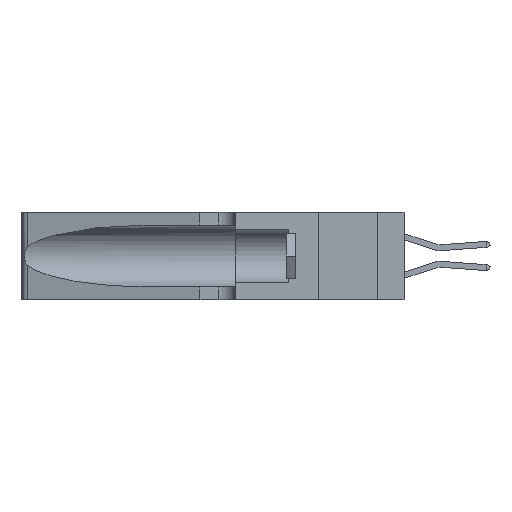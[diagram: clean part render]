
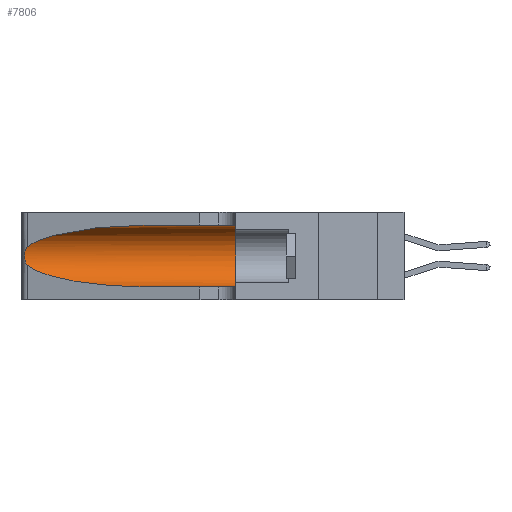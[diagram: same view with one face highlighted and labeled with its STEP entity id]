
A CAD part, left-side view. The second image highlights one B-rep face of the part: STEP entity #7806.
In plain terms, the highlighted cylindrical face has radius 3.308 mm (diameter 6.617 mm), a partial arc.
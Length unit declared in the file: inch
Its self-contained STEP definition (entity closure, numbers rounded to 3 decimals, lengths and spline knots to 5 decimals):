
#732 = DIRECTION ( 'NONE',  ( 0., 1., 0. ) ) ;
#754 = CARTESIAN_POINT ( 'NONE',  ( 0.1305, 0.72297, 0.05475 ) ) ;
#966 = CARTESIAN_POINT ( 'NONE',  ( 0.1305, 0.35, 0.31525 ) ) ;
#1230 = EDGE_CURVE ( 'NONE', #27923, #3265, #6271, .T. ) ;
#1282 = EDGE_CURVE ( 'NONE', #16083, #21831, #34458, .T. ) ;
#2385 =( BOUNDED_CURVE ( )  B_SPLINE_CURVE ( 3, ( #18711, #34994, #7792, #26921 ),
 .UNSPECIFIED., .F., .F. ) 
 B_SPLINE_CURVE_WITH_KNOTS ( ( 4, 4 ),
 ( 1.5708, 2.84003 ),
 .UNSPECIFIED. ) 
 CURVE ( )  GEOMETRIC_REPRESENTATION_ITEM ( )  RATIONAL_B_SPLINE_CURVE ( ( 1., 0.87, 0.87, 1. ) ) 
 REPRESENTATION_ITEM ( '' )  );
#3265 = VERTEX_POINT ( 'NONE', #14024 ) ;
#3901 = CARTESIAN_POINT ( 'NONE',  ( 0.25787, 1.23484, 0.2124 ) ) ;
#4734 = FACE_OUTER_BOUND ( 'NONE', #21937, .T. ) ;
#5455 = VERTEX_POINT ( 'NONE', #12333 ) ;
#5856 = ORIENTED_EDGE ( 'NONE', *, *, #14432, .T. ) ;
#6271 = LINE ( 'NONE', #33257, #12758 ) ;
#6615 = CARTESIAN_POINT ( 'NONE',  ( 0.26018, 1.23835, 0.19895 ) ) ;
#7516 = EDGE_CURVE ( 'NONE', #21831, #3265, #35022, .T. ) ;
#7792 = CARTESIAN_POINT ( 'NONE',  ( 0.2373, 1.15595, 0.28018 ) ) ;
#7806 = ADVANCED_FACE ( 'NONE', ( #4734 ), #18426, .F. ) ;
#8957 = CARTESIAN_POINT ( 'NONE',  ( 0.1305, 1.61858, 0.31525 ) ) ;
#9078 = ORIENTED_EDGE ( 'NONE', *, *, #21233, .T. ) ;
#9411 = CARTESIAN_POINT ( 'NONE',  ( 0.26075, 1.23896, 0.178 ) ) ;
#9803 = CARTESIAN_POINT ( 'NONE',  ( 0.25487, 1.22718, 0.14631 ) ) ;
#12179 = CARTESIAN_POINT ( 'NONE',  ( 0.25856, 1.23593, 0.16098 ) ) ;
#12333 = CARTESIAN_POINT ( 'NONE',  ( 0.25487, 1.22718, 0.22369 ) ) ;
#12522 = B_SPLINE_CURVE_WITH_KNOTS ( 'NONE', 3,
 ( #33800, #14803, #20250, #3901, #23009, #6615, #25760, #9411, #28487, #12179, #31210, #14924, #33919, #17688 ),
 .UNSPECIFIED., .F., .F.,
 ( 4, 2, 2, 2, 2, 2, 4 ),
 ( 0., 0.00027, 0.00053, 0.00107, 0.0016, 0.00187, 0.00214 ),
 .UNSPECIFIED. ) ;
#12758 = VECTOR ( 'NONE', #19810, 39.37008 ) ;
#14024 = CARTESIAN_POINT ( 'NONE',  ( 0.1305, 0.35, 0.05475 ) ) ;
#14432 = EDGE_CURVE ( 'NONE', #16083, #5455, #2385, .T. ) ;
#14803 = CARTESIAN_POINT ( 'NONE',  ( 0.25555, 1.22994, 0.2215 ) ) ;
#14924 = CARTESIAN_POINT ( 'NONE',  ( 0.25639, 1.23186, 0.15144 ) ) ;
#15483 = DIRECTION ( 'NONE',  ( 0., 0., -1. ) ) ;
#16035 = ORIENTED_EDGE ( 'NONE', *, *, #17058, .T. ) ;
#16083 = VERTEX_POINT ( 'NONE', #19166 ) ;
#16690 = ORIENTED_EDGE ( 'NONE', *, *, #1282, .F. ) ;
#16814 = ORIENTED_EDGE ( 'NONE', *, *, #1230, .T. ) ;
#17058 = EDGE_CURVE ( 'NONE', #26505, #27923, #31476, .T. ) ;
#17178 = CARTESIAN_POINT ( 'NONE',  ( 0.1305, 0.35, 0.185 ) ) ;
#17688 = CARTESIAN_POINT ( 'NONE',  ( 0.25487, 1.22718, 0.14631 ) ) ;
#17956 = CARTESIAN_POINT ( 'NONE',  ( 0.18966, 0.96281, 0.05475 ) ) ;
#18426 = CYLINDRICAL_SURFACE ( 'NONE', #27616, 0.13025 ) ;
#18711 = CARTESIAN_POINT ( 'NONE',  ( 0.1305, 0.72297, 0.31525 ) ) ;
#19166 = CARTESIAN_POINT ( 'NONE',  ( 0.1305, 0.72297, 0.31525 ) ) ;
#19810 = DIRECTION ( 'NONE',  ( 0., -1., 0. ) ) ;
#19868 = DIRECTION ( 'NONE',  ( 0., 0., 1. ) ) ;
#20250 = CARTESIAN_POINT ( 'NONE',  ( 0.25639, 1.23184, 0.21858 ) ) ;
#21233 = EDGE_CURVE ( 'NONE', #5455, #26505, #12522, .T. ) ;
#21831 = VERTEX_POINT ( 'NONE', #966 ) ;
#21937 = EDGE_LOOP ( 'NONE', ( #5856, #9078, #16035, #16814, #25113, #16690 ) ) ;
#23009 = CARTESIAN_POINT ( 'NONE',  ( 0.25854, 1.2359, 0.20912 ) ) ;
#23416 = CARTESIAN_POINT ( 'NONE',  ( 0.2373, 1.15595, 0.08982 ) ) ;
#25113 = ORIENTED_EDGE ( 'NONE', *, *, #7516, .F. ) ;
#25423 = DIRECTION ( 'NONE',  ( 0., -1., 0. ) ) ;
#25530 = VECTOR ( 'NONE', #25423, 39.37008 ) ;
#25760 = CARTESIAN_POINT ( 'NONE',  ( 0.26075, 1.23896, 0.19203 ) ) ;
#26319 = DIRECTION ( 'NONE',  ( 0., -1., 0. ) ) ;
#26505 = VERTEX_POINT ( 'NONE', #32299 ) ;
#26921 = CARTESIAN_POINT ( 'NONE',  ( 0.25487, 1.22718, 0.22369 ) ) ;
#27616 = AXIS2_PLACEMENT_3D ( 'NONE', #31754, #26319, #15483 ) ;
#27923 = VERTEX_POINT ( 'NONE', #754 ) ;
#28487 = CARTESIAN_POINT ( 'NONE',  ( 0.26017, 1.23833, 0.17102 ) ) ;
#28872 = CARTESIAN_POINT ( 'NONE',  ( 0.1305, 0.72297, 0.05475 ) ) ;
#30110 = AXIS2_PLACEMENT_3D ( 'NONE', #17178, #732, #19868 ) ;
#31210 = CARTESIAN_POINT ( 'NONE',  ( 0.25789, 1.23486, 0.15765 ) ) ;
#31476 =( BOUNDED_CURVE ( )  B_SPLINE_CURVE ( 3, ( #9803, #23416, #17956, #28872 ),
 .UNSPECIFIED., .F., .T. ) 
 B_SPLINE_CURVE_WITH_KNOTS ( ( 4, 4 ),
 ( 3.44316, 4.71239 ),
 .UNSPECIFIED. ) 
 CURVE ( )  GEOMETRIC_REPRESENTATION_ITEM ( )  RATIONAL_B_SPLINE_CURVE ( ( 1., 0.87, 0.87, 1. ) ) 
 REPRESENTATION_ITEM ( '' )  );
#31754 = CARTESIAN_POINT ( 'NONE',  ( 0.1305, 1.61858, 0.185 ) ) ;
#32299 = CARTESIAN_POINT ( 'NONE',  ( 0.25487, 1.22718, 0.14631 ) ) ;
#33257 = CARTESIAN_POINT ( 'NONE',  ( 0.1305, 1.61858, 0.05475 ) ) ;
#33800 = CARTESIAN_POINT ( 'NONE',  ( 0.25487, 1.22718, 0.22369 ) ) ;
#33919 = CARTESIAN_POINT ( 'NONE',  ( 0.25555, 1.22993, 0.14849 ) ) ;
#34458 = LINE ( 'NONE', #8957, #25530 ) ;
#34994 = CARTESIAN_POINT ( 'NONE',  ( 0.18966, 0.96281, 0.31525 ) ) ;
#35022 = CIRCLE ( 'NONE', #30110, 0.13025 ) ;
